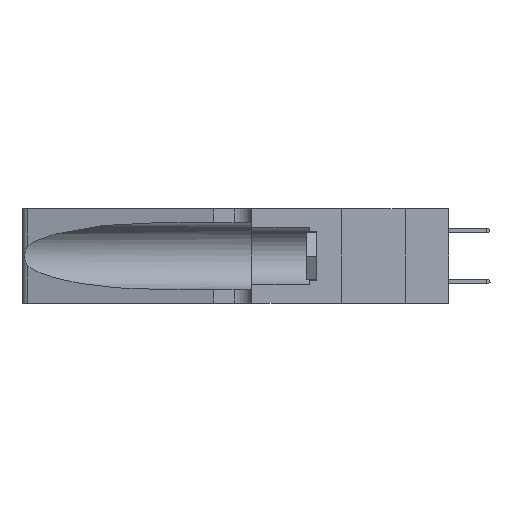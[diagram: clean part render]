
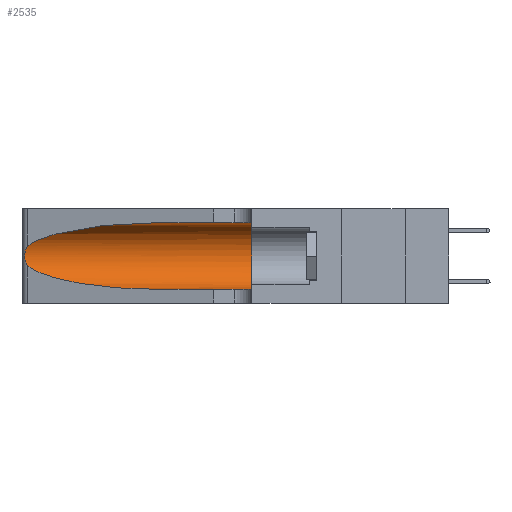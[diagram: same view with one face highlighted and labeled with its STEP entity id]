
A CAD part, left-side view. The second image highlights one B-rep face of the part: STEP entity #2535.
In plain terms, the highlighted cylindrical face has radius 3.308 mm (diameter 6.617 mm), a partial arc.
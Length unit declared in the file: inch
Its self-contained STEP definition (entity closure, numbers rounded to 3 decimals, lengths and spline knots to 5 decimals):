
#99 = CARTESIAN_POINT ( 'NONE',  ( 0.1305, 0.72297, 0.31525 ) ) ;
#300 = CARTESIAN_POINT ( 'NONE',  ( 0.2373, 1.15595, 0.28018 ) ) ;
#864 = EDGE_CURVE ( 'NONE', #10263, #24285, #18752, .T. ) ;
#1153 = CARTESIAN_POINT ( 'NONE',  ( 0.1305, 1.61858, 0.185 ) ) ;
#2535 = ADVANCED_FACE ( 'NONE', ( #25404 ), #13512, .F. ) ;
#3139 = CARTESIAN_POINT ( 'NONE',  ( 0.26018, 1.23835, 0.19895 ) ) ;
#3300 = CARTESIAN_POINT ( 'NONE',  ( 0.2373, 1.15595, 0.08982 ) ) ;
#3588 = ORIENTED_EDGE ( 'NONE', *, *, #8709, .T. ) ;
#4072 = EDGE_LOOP ( 'NONE', ( #14401, #11094, #3588, #19778, #23398, #5305 ) ) ;
#4983 = DIRECTION ( 'NONE',  ( 0., -1., 0. ) ) ;
#5305 = ORIENTED_EDGE ( 'NONE', *, *, #29934, .F. ) ;
#5662 = CARTESIAN_POINT ( 'NONE',  ( 0.25856, 1.23593, 0.16098 ) ) ;
#5769 = CARTESIAN_POINT ( 'NONE',  ( 0.25487, 1.22718, 0.14631 ) ) ;
#6254 = DIRECTION ( 'NONE',  ( 0., -1., 0. ) ) ;
#7636 = LINE ( 'NONE', #17355, #11582 ) ;
#8222 = CARTESIAN_POINT ( 'NONE',  ( 0.25639, 1.23186, 0.15144 ) ) ;
#8709 = EDGE_CURVE ( 'NONE', #29282, #21199, #27685, .T. ) ;
#9137 = DIRECTION ( 'NONE',  ( 0., 1., 0. ) ) ;
#10263 = VERTEX_POINT ( 'NONE', #29377 ) ;
#10425 = CARTESIAN_POINT ( 'NONE',  ( 0.25487, 1.22718, 0.22369 ) ) ;
#10636 = CARTESIAN_POINT ( 'NONE',  ( 0.25787, 1.23484, 0.2124 ) ) ;
#10745 = CARTESIAN_POINT ( 'NONE',  ( 0.25555, 1.22993, 0.14849 ) ) ;
#10968 = CARTESIAN_POINT ( 'NONE',  ( 0.25555, 1.22994, 0.2215 ) ) ;
#11032 = CARTESIAN_POINT ( 'NONE',  ( 0.18966, 0.96281, 0.05475 ) ) ;
#11094 = ORIENTED_EDGE ( 'NONE', *, *, #32175, .T. ) ;
#11269 = VERTEX_POINT ( 'NONE', #14994 ) ;
#11275 = CARTESIAN_POINT ( 'NONE',  ( 0.25487, 1.22718, 0.14631 ) ) ;
#11582 = VECTOR ( 'NONE', #4983, 39.37008 ) ;
#13072 = B_SPLINE_CURVE_WITH_KNOTS ( 'NONE', 3,
 ( #26009, #10968, #13627, #10636, #28550, #3139, #28337, #15707, #28653, #5662, #23375, #8222, #10745, #5769 ),
 .UNSPECIFIED., .F., .F.,
 ( 4, 2, 2, 2, 2, 2, 4 ),
 ( 0., 0.00027, 0.00053, 0.00107, 0.0016, 0.00187, 0.00214 ),
 .UNSPECIFIED. ) ;
#13512 = CYLINDRICAL_SURFACE ( 'NONE', #25049, 0.13025 ) ;
#13627 = CARTESIAN_POINT ( 'NONE',  ( 0.25639, 1.23184, 0.21858 ) ) ;
#13971 = AXIS2_PLACEMENT_3D ( 'NONE', #24512, #9137, #31900 ) ;
#14401 = ORIENTED_EDGE ( 'NONE', *, *, #21653, .T. ) ;
#14994 = CARTESIAN_POINT ( 'NONE',  ( 0.25487, 1.22718, 0.22369 ) ) ;
#15406 = CARTESIAN_POINT ( 'NONE',  ( 0.18966, 0.96281, 0.31525 ) ) ;
#15707 = CARTESIAN_POINT ( 'NONE',  ( 0.26075, 1.23896, 0.178 ) ) ;
#16215 = CARTESIAN_POINT ( 'NONE',  ( 0.1305, 0.72297, 0.05475 ) ) ;
#16255 = DIRECTION ( 'NONE',  ( 0., 0., -1. ) ) ;
#17355 = CARTESIAN_POINT ( 'NONE',  ( 0.1305, 1.61858, 0.05475 ) ) ;
#18526 =( BOUNDED_CURVE ( )  B_SPLINE_CURVE ( 3, ( #30570, #15406, #300, #10425 ),
 .UNSPECIFIED., .F., .F. ) 
 B_SPLINE_CURVE_WITH_KNOTS ( ( 4, 4 ),
 ( 1.5708, 2.84003 ),
 .UNSPECIFIED. ) 
 CURVE ( )  GEOMETRIC_REPRESENTATION_ITEM ( )  RATIONAL_B_SPLINE_CURVE ( ( 1., 0.87, 0.87, 1. ) ) 
 REPRESENTATION_ITEM ( '' )  );
#18746 = CARTESIAN_POINT ( 'NONE',  ( 0.25487, 1.22718, 0.14631 ) ) ;
#18752 = CIRCLE ( 'NONE', #13971, 0.13025 ) ;
#18842 = CARTESIAN_POINT ( 'NONE',  ( 0.1305, 1.61858, 0.31525 ) ) ;
#18909 = CARTESIAN_POINT ( 'NONE',  ( 0.1305, 0.35, 0.05475 ) ) ;
#19778 = ORIENTED_EDGE ( 'NONE', *, *, #32529, .T. ) ;
#20911 = VECTOR ( 'NONE', #6254, 39.37008 ) ;
#21199 = VERTEX_POINT ( 'NONE', #31787 ) ;
#21653 = EDGE_CURVE ( 'NONE', #27252, #11269, #18526, .T. ) ;
#23375 = CARTESIAN_POINT ( 'NONE',  ( 0.25789, 1.23486, 0.15765 ) ) ;
#23398 = ORIENTED_EDGE ( 'NONE', *, *, #864, .F. ) ;
#24285 = VERTEX_POINT ( 'NONE', #18909 ) ;
#24512 = CARTESIAN_POINT ( 'NONE',  ( 0.1305, 0.35, 0.185 ) ) ;
#25049 = AXIS2_PLACEMENT_3D ( 'NONE', #1153, #31293, #16255 ) ;
#25404 = FACE_OUTER_BOUND ( 'NONE', #4072, .T. ) ;
#26009 = CARTESIAN_POINT ( 'NONE',  ( 0.25487, 1.22718, 0.22369 ) ) ;
#27252 = VERTEX_POINT ( 'NONE', #99 ) ;
#27685 =( BOUNDED_CURVE ( )  B_SPLINE_CURVE ( 3, ( #18746, #3300, #11032, #16215 ),
 .UNSPECIFIED., .F., .F. ) 
 B_SPLINE_CURVE_WITH_KNOTS ( ( 4, 4 ),
 ( 3.44316, 4.71239 ),
 .UNSPECIFIED. ) 
 CURVE ( )  GEOMETRIC_REPRESENTATION_ITEM ( )  RATIONAL_B_SPLINE_CURVE ( ( 1., 0.87, 0.87, 1. ) ) 
 REPRESENTATION_ITEM ( '' )  );
#28337 = CARTESIAN_POINT ( 'NONE',  ( 0.26075, 1.23896, 0.19203 ) ) ;
#28550 = CARTESIAN_POINT ( 'NONE',  ( 0.25854, 1.2359, 0.20912 ) ) ;
#28653 = CARTESIAN_POINT ( 'NONE',  ( 0.26017, 1.23833, 0.17102 ) ) ;
#29282 = VERTEX_POINT ( 'NONE', #11275 ) ;
#29377 = CARTESIAN_POINT ( 'NONE',  ( 0.1305, 0.35, 0.31525 ) ) ;
#29934 = EDGE_CURVE ( 'NONE', #27252, #10263, #32031, .T. ) ;
#30570 = CARTESIAN_POINT ( 'NONE',  ( 0.1305, 0.72297, 0.31525 ) ) ;
#31293 = DIRECTION ( 'NONE',  ( 0., -1., 0. ) ) ;
#31787 = CARTESIAN_POINT ( 'NONE',  ( 0.1305, 0.72297, 0.05475 ) ) ;
#31900 = DIRECTION ( 'NONE',  ( 0., 0., 1. ) ) ;
#32031 = LINE ( 'NONE', #18842, #20911 ) ;
#32175 = EDGE_CURVE ( 'NONE', #11269, #29282, #13072, .T. ) ;
#32529 = EDGE_CURVE ( 'NONE', #21199, #24285, #7636, .T. ) ;
